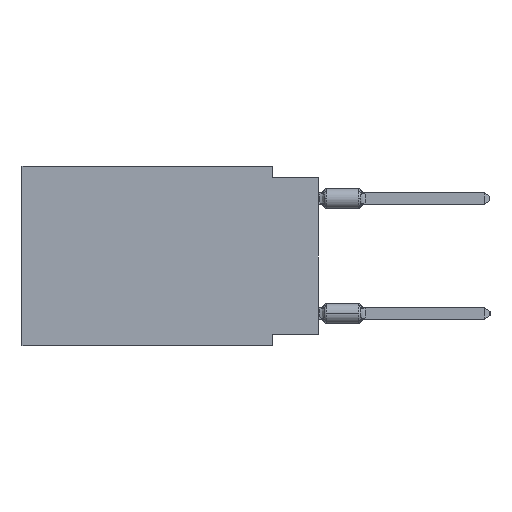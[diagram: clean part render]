
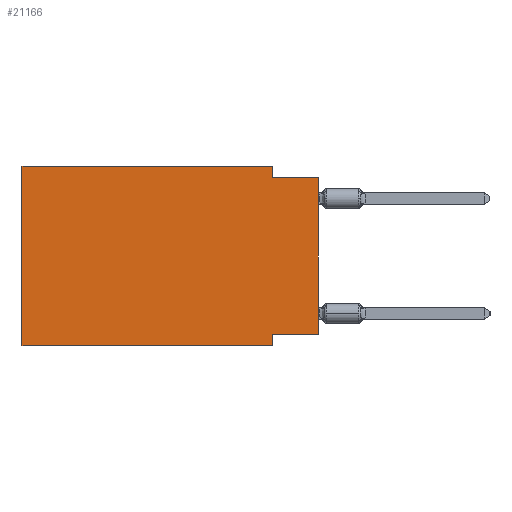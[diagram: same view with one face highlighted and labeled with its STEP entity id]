
A CAD part, left-side view. The second image highlights one B-rep face of the part: STEP entity #21166.
In plain terms, the highlighted planar face has unit normal (-1, 0, 0).
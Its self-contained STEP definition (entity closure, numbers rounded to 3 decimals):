
#248 = VECTOR ( 'NONE', #21852, 1000. ) ;
#707 = EDGE_LOOP ( 'NONE', ( #15676, #5377, #52903, #26017, #45415, #22254, #24357, #22325 ) ) ;
#3339 = LINE ( 'NONE', #43571, #42477 ) ;
#3547 = VERTEX_POINT ( 'NONE', #29530 ) ;
#4690 = DIRECTION ( 'NONE',  ( 0., -1., 0. ) ) ;
#4935 = EDGE_CURVE ( 'NONE', #37820, #22465, #49487, .T. ) ;
#5377 = ORIENTED_EDGE ( 'NONE', *, *, #24399, .F. ) ;
#5741 = PLANE ( 'NONE',  #36638 ) ;
#6008 = VECTOR ( 'NONE', #44086, 1000. ) ;
#6925 = DIRECTION ( 'NONE',  ( 0., 0., 1. ) ) ;
#7323 = EDGE_CURVE ( 'NONE', #37655, #3547, #49626, .T. ) ;
#8739 = DIRECTION ( 'NONE',  ( 0., 0., -1. ) ) ;
#9846 = CARTESIAN_POINT ( 'NONE',  ( 0., 2.54, 0. ) ) ;
#10575 = CARTESIAN_POINT ( 'NONE',  ( 0., 0., -0.635 ) ) ;
#11372 = CARTESIAN_POINT ( 'NONE',  ( 0., 16.383, -9.906 ) ) ;
#13894 = VECTOR ( 'NONE', #4690, 1000. ) ;
#15676 = ORIENTED_EDGE ( 'NONE', *, *, #4935, .T. ) ;
#15706 = CARTESIAN_POINT ( 'NONE',  ( 0., 16.383, 0. ) ) ;
#16075 = VERTEX_POINT ( 'NONE', #55456 ) ;
#16562 = VECTOR ( 'NONE', #6925, 1000. ) ;
#18408 = LINE ( 'NONE', #9846, #248 ) ;
#18565 = DIRECTION ( 'NONE',  ( 0., 0., -1. ) ) ;
#20310 = CARTESIAN_POINT ( 'NONE',  ( 0., 16.383, -9.906 ) ) ;
#20511 = EDGE_CURVE ( 'NONE', #33118, #25851, #33822, .T. ) ;
#21166 = ADVANCED_FACE ( 'NONE', ( #31976 ), #5741, .F. ) ;
#21852 = DIRECTION ( 'NONE',  ( 0., 0., -1. ) ) ;
#22254 = ORIENTED_EDGE ( 'NONE', *, *, #7323, .T. ) ;
#22325 = ORIENTED_EDGE ( 'NONE', *, *, #46447, .F. ) ;
#22465 = VERTEX_POINT ( 'NONE', #10575 ) ;
#22603 = LINE ( 'NONE', #30414, #22953 ) ;
#22953 = VECTOR ( 'NONE', #47846, 1000. ) ;
#24115 = CARTESIAN_POINT ( 'NONE',  ( 0., 2.54, -9.271 ) ) ;
#24357 = ORIENTED_EDGE ( 'NONE', *, *, #32016, .F. ) ;
#24399 = EDGE_CURVE ( 'NONE', #16075, #22465, #32986, .T. ) ;
#25851 = VERTEX_POINT ( 'NONE', #51577 ) ;
#26017 = ORIENTED_EDGE ( 'NONE', *, *, #20511, .F. ) ;
#26832 = VECTOR ( 'NONE', #28118, 1000. ) ;
#28118 = DIRECTION ( 'NONE',  ( 0., -1., 0. ) ) ;
#28773 = DIRECTION ( 'NONE',  ( 0., -1., 0. ) ) ;
#29530 = CARTESIAN_POINT ( 'NONE',  ( 0., 2.54, -9.906 ) ) ;
#30414 = CARTESIAN_POINT ( 'NONE',  ( 0., 0., -9.271 ) ) ;
#31976 = FACE_OUTER_BOUND ( 'NONE', #707, .T. ) ;
#32016 = EDGE_CURVE ( 'NONE', #47786, #3547, #3339, .T. ) ;
#32596 = LINE ( 'NONE', #50018, #16562 ) ;
#32986 = LINE ( 'NONE', #50411, #26832 ) ;
#33118 = VERTEX_POINT ( 'NONE', #15706 ) ;
#33822 = LINE ( 'NONE', #51238, #13894 ) ;
#34557 = CARTESIAN_POINT ( 'NONE',  ( 0., 0., -9.271 ) ) ;
#36264 = DIRECTION ( 'NONE',  ( 1., 0., 0. ) ) ;
#36638 = AXIS2_PLACEMENT_3D ( 'NONE', #53412, #36264, #18565 ) ;
#37655 = VERTEX_POINT ( 'NONE', #20310 ) ;
#37820 = VERTEX_POINT ( 'NONE', #34557 ) ;
#41778 = VECTOR ( 'NONE', #28773, 1000. ) ;
#42477 = VECTOR ( 'NONE', #8739, 1000. ) ;
#43571 = CARTESIAN_POINT ( 'NONE',  ( 0., 2.54, -9.906 ) ) ;
#44086 = DIRECTION ( 'NONE',  ( 0., 0., 1. ) ) ;
#44641 = CARTESIAN_POINT ( 'NONE',  ( 0., 0., 0. ) ) ;
#45415 = ORIENTED_EDGE ( 'NONE', *, *, #46577, .F. ) ;
#46447 = EDGE_CURVE ( 'NONE', #37820, #47786, #22603, .T. ) ;
#46577 = EDGE_CURVE ( 'NONE', #37655, #33118, #32596, .T. ) ;
#47651 = EDGE_CURVE ( 'NONE', #25851, #16075, #18408, .T. ) ;
#47786 = VERTEX_POINT ( 'NONE', #24115 ) ;
#47846 = DIRECTION ( 'NONE',  ( 0., 1., 0. ) ) ;
#49487 = LINE ( 'NONE', #44641, #6008 ) ;
#49626 = LINE ( 'NONE', #11372, #41778 ) ;
#50018 = CARTESIAN_POINT ( 'NONE',  ( 0., 16.383, 0. ) ) ;
#50411 = CARTESIAN_POINT ( 'NONE',  ( 0., 0., -0.635 ) ) ;
#51238 = CARTESIAN_POINT ( 'NONE',  ( 0., 16.383, 0. ) ) ;
#51577 = CARTESIAN_POINT ( 'NONE',  ( 0., 2.54, 0. ) ) ;
#52903 = ORIENTED_EDGE ( 'NONE', *, *, #47651, .F. ) ;
#53412 = CARTESIAN_POINT ( 'NONE',  ( 0., 16.383, 0. ) ) ;
#55456 = CARTESIAN_POINT ( 'NONE',  ( 0., 2.54, -0.635 ) ) ;
